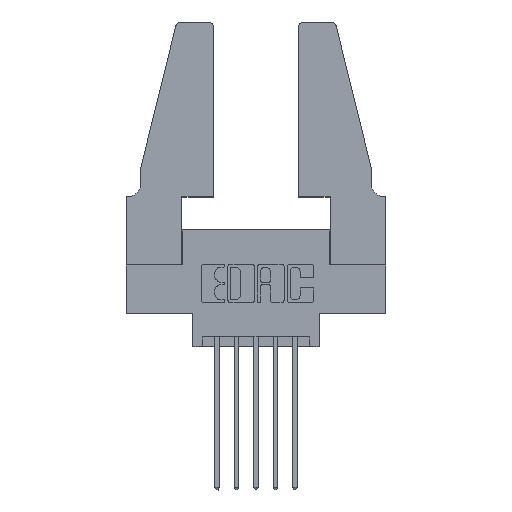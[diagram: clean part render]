
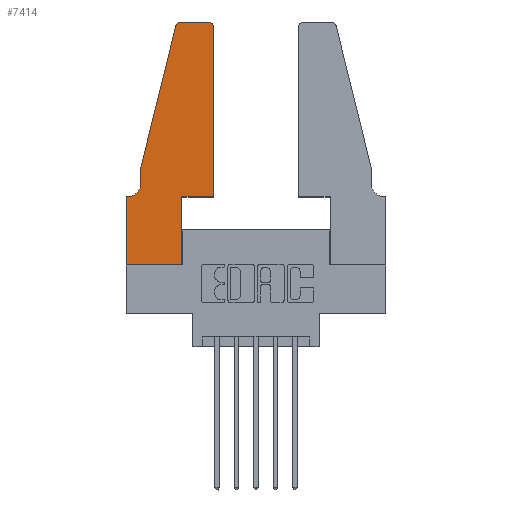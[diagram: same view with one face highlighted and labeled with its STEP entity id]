
A CAD part, top view. The second image highlights one B-rep face of the part: STEP entity #7414.
In plain terms, the highlighted planar face has unit normal (0, 0, 1).
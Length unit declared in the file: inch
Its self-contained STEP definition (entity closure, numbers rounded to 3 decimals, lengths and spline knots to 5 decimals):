
#76 = EDGE_CURVE ( 'NONE', #9242, #4929, #1084, .T. ) ;
#201 = DIRECTION ( 'NONE',  ( 1., 0., 0. ) ) ;
#286 = ORIENTED_EDGE ( 'NONE', *, *, #2326, .T. ) ;
#438 = ORIENTED_EDGE ( 'NONE', *, *, #76, .T. ) ;
#550 = DIRECTION ( 'NONE',  ( -0.239, -0.971, 0. ) ) ;
#710 = DIRECTION ( 'NONE',  ( 0., 1., 0. ) ) ;
#840 = DIRECTION ( 'NONE',  ( 0., 0., -1. ) ) ;
#926 = EDGE_CURVE ( 'NONE', #9750, #8751, #2145, .T. ) ;
#999 = CARTESIAN_POINT ( 'NONE',  ( 0.4505, 0.35, 0.37 ) ) ;
#1084 = LINE ( 'NONE', #6885, #9781 ) ;
#1094 = VERTEX_POINT ( 'NONE', #2950 ) ;
#1227 = DIRECTION ( 'NONE',  ( -1., 0., 0. ) ) ;
#1265 = VERTEX_POINT ( 'NONE', #7440 ) ;
#1276 = VECTOR ( 'NONE', #7706, 39.37008 ) ;
#1554 = CARTESIAN_POINT ( 'NONE',  ( 0.0755, 0.35, 0.37 ) ) ;
#1678 = CARTESIAN_POINT ( 'NONE',  ( 0., 0., 0.37 ) ) ;
#2140 = CARTESIAN_POINT ( 'NONE',  ( 0.2605, 1.25, 0.37 ) ) ;
#2145 = CIRCLE ( 'NONE', #5284, 0.03 ) ;
#2308 = CARTESIAN_POINT ( 'NONE',  ( 0., 0.35, 0.37 ) ) ;
#2326 = EDGE_CURVE ( 'NONE', #8751, #9242, #4152, .T. ) ;
#2753 = LINE ( 'NONE', #2140, #9420 ) ;
#2792 = CARTESIAN_POINT ( 'NONE',  ( 0., 0., 0.37 ) ) ;
#2947 = CARTESIAN_POINT ( 'NONE',  ( 0.2865, 0.35, 0.37 ) ) ;
#2950 = CARTESIAN_POINT ( 'NONE',  ( 0.2865, 0.35, 0.37 ) ) ;
#3166 = DIRECTION ( 'NONE',  ( 0., 0., 1. ) ) ;
#3203 = PLANE ( 'NONE',  #10433 ) ;
#3748 = DIRECTION ( 'NONE',  ( 0., 1., 0. ) ) ;
#3832 = EDGE_CURVE ( 'NONE', #1265, #9750, #2753, .T. ) ;
#3880 = ORIENTED_EDGE ( 'NONE', *, *, #5187, .T. ) ;
#4005 = VERTEX_POINT ( 'NONE', #4232 ) ;
#4075 = EDGE_CURVE ( 'NONE', #4990, #1094, #10762, .T. ) ;
#4093 = ORIENTED_EDGE ( 'NONE', *, *, #6974, .T. ) ;
#4152 = LINE ( 'NONE', #4828, #4842 ) ;
#4167 = CARTESIAN_POINT ( 'NONE',  ( 0.4505, 0.35, 0.37 ) ) ;
#4232 = CARTESIAN_POINT ( 'NONE',  ( 0., 0.35, 0.37 ) ) ;
#4272 = DIRECTION ( 'NONE',  ( 0., 0., 1. ) ) ;
#4302 = CARTESIAN_POINT ( 'NONE',  ( 0.284, 1.25, 0.37 ) ) ;
#4426 = CARTESIAN_POINT ( 'NONE',  ( 0., 0., 0.37 ) ) ;
#4447 = EDGE_CURVE ( 'NONE', #9991, #7334, #10892, .T. ) ;
#4828 = CARTESIAN_POINT ( 'NONE',  ( 0.0755, 0.5, 0.37 ) ) ;
#4842 = VECTOR ( 'NONE', #550, 39.37008 ) ;
#4855 = VECTOR ( 'NONE', #201, 39.37008 ) ;
#4929 = VERTEX_POINT ( 'NONE', #8176 ) ;
#4990 = VERTEX_POINT ( 'NONE', #8289 ) ;
#5187 = EDGE_CURVE ( 'NONE', #1094, #9991, #6620, .T. ) ;
#5284 = AXIS2_PLACEMENT_3D ( 'NONE', #7737, #4272, #8597 ) ;
#5364 = DIRECTION ( 'NONE',  ( -1., 0., 0. ) ) ;
#5422 = AXIS2_PLACEMENT_3D ( 'NONE', #7047, #840, #5364 ) ;
#5528 = ORIENTED_EDGE ( 'NONE', *, *, #926, .T. ) ;
#5546 = CARTESIAN_POINT ( 'NONE',  ( 0.0755, 0.5, 0.37 ) ) ;
#5651 = VECTOR ( 'NONE', #3748, 39.37008 ) ;
#5868 = ORIENTED_EDGE ( 'NONE', *, *, #4447, .T. ) ;
#5932 = LINE ( 'NONE', #2792, #1276 ) ;
#5993 = DIRECTION ( 'NONE',  ( 1., 0., 0. ) ) ;
#6034 = LINE ( 'NONE', #1678, #7111 ) ;
#6037 = DIRECTION ( 'NONE',  ( -1., 0., 0. ) ) ;
#6106 = DIRECTION ( 'NONE',  ( 0., -1., 0. ) ) ;
#6117 = CIRCLE ( 'NONE', #5422, 0.07 ) ;
#6176 = ORIENTED_EDGE ( 'NONE', *, *, #4075, .T. ) ;
#6310 = VECTOR ( 'NONE', #710, 39.37008 ) ;
#6584 = FACE_OUTER_BOUND ( 'NONE', #8497, .T. ) ;
#6620 = LINE ( 'NONE', #999, #4855 ) ;
#6644 = VECTOR ( 'NONE', #6037, 39.37008 ) ;
#6768 = EDGE_CURVE ( 'NONE', #4005, #8755, #5932, .T. ) ;
#6885 = CARTESIAN_POINT ( 'NONE',  ( 0.0755, 0.5, 0.37 ) ) ;
#6974 = EDGE_CURVE ( 'NONE', #7334, #1265, #10486, .T. ) ;
#7004 = ORIENTED_EDGE ( 'NONE', *, *, #9618, .T. ) ;
#7047 = CARTESIAN_POINT ( 'NONE',  ( 0.0055, 0.42, 0.37 ) ) ;
#7111 = VECTOR ( 'NONE', #8701, 39.37008 ) ;
#7334 = VERTEX_POINT ( 'NONE', #9815 ) ;
#7414 = ADVANCED_FACE ( 'NONE', ( #6584 ), #3203, .T. ) ;
#7440 = CARTESIAN_POINT ( 'NONE',  ( 0.4205, 1.25, 0.37 ) ) ;
#7578 = EDGE_CURVE ( 'NONE', #8755, #4990, #6034, .T. ) ;
#7706 = DIRECTION ( 'NONE',  ( 0., -1., 0. ) ) ;
#7737 = CARTESIAN_POINT ( 'NONE',  ( 0.284, 1.22, 0.37 ) ) ;
#7889 = ORIENTED_EDGE ( 'NONE', *, *, #10829, .T. ) ;
#8176 = CARTESIAN_POINT ( 'NONE',  ( 0.0755, 0.42, 0.37 ) ) ;
#8289 = CARTESIAN_POINT ( 'NONE',  ( 0.2865, 0., 0.37 ) ) ;
#8497 = EDGE_LOOP ( 'NONE', ( #9934, #5528, #286, #438, #7004, #7889, #9013, #11022, #6176, #3880, #5868, #4093 ) ) ;
#8532 = AXIS2_PLACEMENT_3D ( 'NONE', #9427, #10270, #5993 ) ;
#8574 = CARTESIAN_POINT ( 'NONE',  ( 0.4505, 0.35, 0.37 ) ) ;
#8597 = DIRECTION ( 'NONE',  ( 1., 0., 0. ) ) ;
#8701 = DIRECTION ( 'NONE',  ( 1., 0., 0. ) ) ;
#8751 = VERTEX_POINT ( 'NONE', #8783 ) ;
#8755 = VERTEX_POINT ( 'NONE', #4426 ) ;
#8783 = CARTESIAN_POINT ( 'NONE',  ( 0.25487, 1.22718, 0.37 ) ) ;
#9013 = ORIENTED_EDGE ( 'NONE', *, *, #6768, .T. ) ;
#9242 = VERTEX_POINT ( 'NONE', #5546 ) ;
#9420 = VECTOR ( 'NONE', #1227, 39.37008 ) ;
#9427 = CARTESIAN_POINT ( 'NONE',  ( 0.4205, 1.22, 0.37 ) ) ;
#9568 = CARTESIAN_POINT ( 'NONE',  ( 0.0055, 0.35, 0.37 ) ) ;
#9593 = VERTEX_POINT ( 'NONE', #9568 ) ;
#9612 = LINE ( 'NONE', #1554, #6644 ) ;
#9618 = EDGE_CURVE ( 'NONE', #4929, #9593, #6117, .T. ) ;
#9750 = VERTEX_POINT ( 'NONE', #4302 ) ;
#9781 = VECTOR ( 'NONE', #6106, 39.37008 ) ;
#9815 = CARTESIAN_POINT ( 'NONE',  ( 0.4505, 1.22, 0.37 ) ) ;
#9934 = ORIENTED_EDGE ( 'NONE', *, *, #3832, .T. ) ;
#9991 = VERTEX_POINT ( 'NONE', #8574 ) ;
#10086 = DIRECTION ( 'NONE',  ( 1., 0., 0. ) ) ;
#10270 = DIRECTION ( 'NONE',  ( 0., 0., 1. ) ) ;
#10433 = AXIS2_PLACEMENT_3D ( 'NONE', #2308, #3166, #10086 ) ;
#10486 = CIRCLE ( 'NONE', #8532, 0.03 ) ;
#10762 = LINE ( 'NONE', #2947, #5651 ) ;
#10829 = EDGE_CURVE ( 'NONE', #9593, #4005, #9612, .T. ) ;
#10892 = LINE ( 'NONE', #4167, #6310 ) ;
#11022 = ORIENTED_EDGE ( 'NONE', *, *, #7578, .T. ) ;
